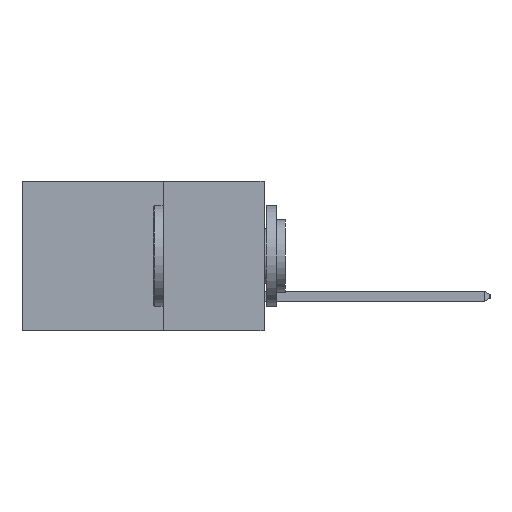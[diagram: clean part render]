
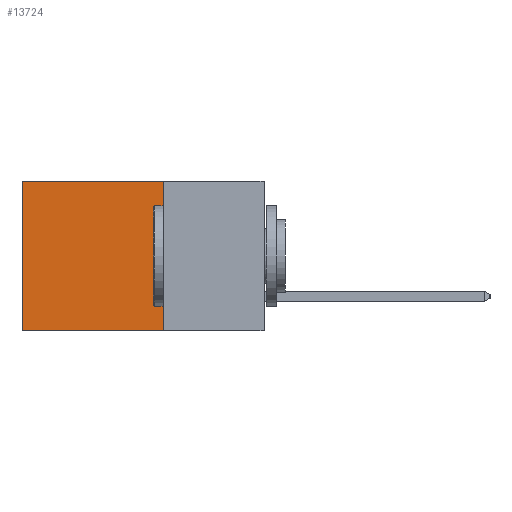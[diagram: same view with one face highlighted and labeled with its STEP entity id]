
A CAD part, left-side view. The second image highlights one B-rep face of the part: STEP entity #13724.
In plain terms, the highlighted planar face has unit normal (-1, 0, 0).
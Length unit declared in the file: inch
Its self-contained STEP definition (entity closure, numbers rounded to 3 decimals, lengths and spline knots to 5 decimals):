
#569 = ORIENTED_EDGE ( 'NONE', *, *, #18076, .F. ) ;
#667 = CARTESIAN_POINT ( 'NONE',  ( 0.298, 0.6, 0. ) ) ;
#902 = VERTEX_POINT ( 'NONE', #16507 ) ;
#1215 = LINE ( 'NONE', #667, #21876 ) ;
#1870 = LINE ( 'NONE', #19672, #11901 ) ;
#3134 = VERTEX_POINT ( 'NONE', #18481 ) ;
#3359 = EDGE_LOOP ( 'NONE', ( #11297, #569, #15006, #19884 ) ) ;
#3365 = CARTESIAN_POINT ( 'NONE',  ( 0.298, 0.25, 0. ) ) ;
#3890 = CARTESIAN_POINT ( 'NONE',  ( 0.298, 0.6, -0.37 ) ) ;
#4710 = DIRECTION ( 'NONE',  ( 0., 0., -1. ) ) ;
#5839 = CARTESIAN_POINT ( 'NONE',  ( 0.298, 0.25, -0.37 ) ) ;
#6201 = PLANE ( 'NONE',  #17813 ) ;
#7723 = VERTEX_POINT ( 'NONE', #3890 ) ;
#8232 = FACE_OUTER_BOUND ( 'NONE', #3359, .T. ) ;
#8654 = VECTOR ( 'NONE', #19862, 39.37008 ) ;
#9713 = DIRECTION ( 'NONE',  ( 0., 1., 0. ) ) ;
#9724 = CARTESIAN_POINT ( 'NONE',  ( 0.298, 0.25, 0. ) ) ;
#10278 = DIRECTION ( 'NONE',  ( 0., 0., -1. ) ) ;
#11297 = ORIENTED_EDGE ( 'NONE', *, *, #15937, .T. ) ;
#11901 = VECTOR ( 'NONE', #9713, 39.37008 ) ;
#13291 = LINE ( 'NONE', #5839, #8654 ) ;
#13724 = ADVANCED_FACE ( 'NONE', ( #8232 ), #6201, .F. ) ;
#14569 = LINE ( 'NONE', #9724, #25057 ) ;
#15006 = ORIENTED_EDGE ( 'NONE', *, *, #18028, .F. ) ;
#15937 = EDGE_CURVE ( 'NONE', #902, #7723, #1215, .T. ) ;
#16507 = CARTESIAN_POINT ( 'NONE',  ( 0.298, 0.6, 0. ) ) ;
#17813 = AXIS2_PLACEMENT_3D ( 'NONE', #20251, #22181, #10278 ) ;
#18028 = EDGE_CURVE ( 'NONE', #23216, #3134, #14569, .T. ) ;
#18076 = EDGE_CURVE ( 'NONE', #3134, #7723, #13291, .T. ) ;
#18481 = CARTESIAN_POINT ( 'NONE',  ( 0.298, 0.25, -0.37 ) ) ;
#19672 = CARTESIAN_POINT ( 'NONE',  ( 0.298, 0.25, 0. ) ) ;
#19862 = DIRECTION ( 'NONE',  ( 0., 1., 0. ) ) ;
#19884 = ORIENTED_EDGE ( 'NONE', *, *, #21331, .T. ) ;
#20251 = CARTESIAN_POINT ( 'NONE',  ( 0.298, 0.25, 0. ) ) ;
#21331 = EDGE_CURVE ( 'NONE', #23216, #902, #1870, .T. ) ;
#21876 = VECTOR ( 'NONE', #4710, 39.37008 ) ;
#22181 = DIRECTION ( 'NONE',  ( 1., 0., 0. ) ) ;
#23216 = VERTEX_POINT ( 'NONE', #3365 ) ;
#25057 = VECTOR ( 'NONE', #25513, 39.37008 ) ;
#25513 = DIRECTION ( 'NONE',  ( 0., 0., -1. ) ) ;
